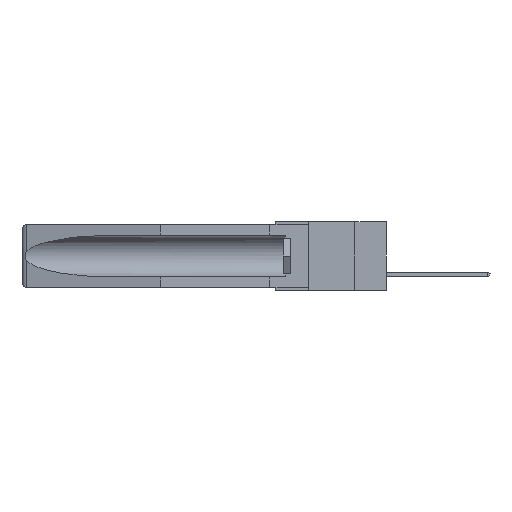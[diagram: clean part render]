
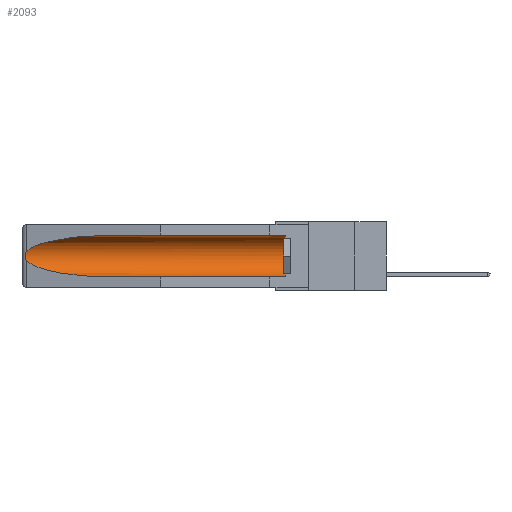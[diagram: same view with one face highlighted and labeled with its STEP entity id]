
A CAD part, left-side view. The second image highlights one B-rep face of the part: STEP entity #2093.
In plain terms, the highlighted cylindrical face has radius 2.857 mm (diameter 5.715 mm), a partial arc.
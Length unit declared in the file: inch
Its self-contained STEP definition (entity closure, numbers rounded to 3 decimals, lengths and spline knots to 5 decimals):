
#7 = CARTESIAN_POINT ( 'NONE',  ( 0.155, 0.126, -0.284 ) ) ;
#338 = CARTESIAN_POINT ( 'NONE',  ( 0.26655, 1.53094, -0.18657 ) ) ;
#1060 = ORIENTED_EDGE ( 'NONE', *, *, #14744, .T. ) ;
#1366 = CARTESIAN_POINT ( 'NONE',  ( 0.155, -0.30754, -0.284 ) ) ;
#1435 = CYLINDRICAL_SURFACE ( 'NONE', #15968, 0.1125 ) ;
#1681 = CARTESIAN_POINT ( 'NONE',  ( 0.155, 0.126, -0.1715 ) ) ;
#1811 = CARTESIAN_POINT ( 'NONE',  ( 0.155, -0.30754, -0.059 ) ) ;
#2093 = ADVANCED_FACE ( 'NONE', ( #4897 ), #1435, .F. ) ;
#2666 = VERTEX_POINT ( 'NONE', #25643 ) ;
#3251 = CARTESIAN_POINT ( 'NONE',  ( 0.21114, 1.30732, -0.059 ) ) ;
#3827 = DIRECTION ( 'NONE',  ( 0., 1., 0. ) ) ;
#3974 = CARTESIAN_POINT ( 'NONE',  ( 0.21114, 1.30732, -0.284 ) ) ;
#4140 = CARTESIAN_POINT ( 'NONE',  ( 0.2675, 1.53308, -0.17534 ) ) ;
#4897 = FACE_OUTER_BOUND ( 'NONE', #23598, .T. ) ;
#5046 = CARTESIAN_POINT ( 'NONE',  ( 0.155, -0.30754, -0.1715 ) ) ;
#5417 = VERTEX_POINT ( 'NONE', #7 ) ;
#7285 = ORIENTED_EDGE ( 'NONE', *, *, #19025, .T. ) ;
#8301 = CARTESIAN_POINT ( 'NONE',  ( 0.2673, 1.53269, -0.17917 ) ) ;
#8381 = CARTESIAN_POINT ( 'NONE',  ( 0.26654, 1.53092, -0.15636 ) ) ;
#8809 = EDGE_CURVE ( 'NONE', #5417, #25534, #17267, .T. ) ;
#8903 =( BOUNDED_CURVE ( )  B_SPLINE_CURVE ( 3, ( #23864, #11619, #3974, #10264 ),
 .UNSPECIFIED., .F., .F. ) 
 B_SPLINE_CURVE_WITH_KNOTS ( ( 4, 4 ),
 ( 0.1948, 1.5708 ),
 .UNSPECIFIED. ) 
 CURVE ( )  GEOMETRIC_REPRESENTATION_ITEM ( )  RATIONAL_B_SPLINE_CURVE ( ( 1., 0.848, 0.848, 1. ) ) 
 REPRESENTATION_ITEM ( '' )  );
#9391 = B_SPLINE_CURVE_WITH_KNOTS ( 'NONE', 3,
 ( #24817, #22938, #8381, #22679, #12441, #4140, #8301, #338, #20899, #10344 ),
 .UNSPECIFIED., .F., .F.,
 ( 4, 2, 2, 2, 4 ),
 ( 0., 0.00029, 0.00058, 0.00087, 0.00117 ),
 .UNSPECIFIED. ) ;
#9770 = CARTESIAN_POINT ( 'NONE',  ( 0.155, 0.126, -0.059 ) ) ;
#10205 =( BOUNDED_CURVE ( )  B_SPLINE_CURVE ( 3, ( #15561, #3251, #25621, #25446 ),
 .UNSPECIFIED., .F., .T. ) 
 B_SPLINE_CURVE_WITH_KNOTS ( ( 4, 4 ),
 ( 4.71239, 6.08839 ),
 .UNSPECIFIED. ) 
 CURVE ( )  GEOMETRIC_REPRESENTATION_ITEM ( )  RATIONAL_B_SPLINE_CURVE ( ( 1., 0.848, 0.848, 1. ) ) 
 REPRESENTATION_ITEM ( '' )  );
#10264 = CARTESIAN_POINT ( 'NONE',  ( 0.155, 1.07973, -0.284 ) ) ;
#10344 = CARTESIAN_POINT ( 'NONE',  ( 0.26537, 1.52718, -0.19328 ) ) ;
#10730 = VECTOR ( 'NONE', #3827, 39.37008 ) ;
#11619 = CARTESIAN_POINT ( 'NONE',  ( 0.25451, 1.48313, -0.24835 ) ) ;
#11975 = DIRECTION ( 'NONE',  ( 0., 1., 0. ) ) ;
#12441 = CARTESIAN_POINT ( 'NONE',  ( 0.2675, 1.53308, -0.16763 ) ) ;
#12499 = VERTEX_POINT ( 'NONE', #17276 ) ;
#13104 = EDGE_CURVE ( 'NONE', #5417, #16220, #15054, .T. ) ;
#13643 = ORIENTED_EDGE ( 'NONE', *, *, #16625, .T. ) ;
#13783 = VECTOR ( 'NONE', #25931, 39.37008 ) ;
#14066 = DIRECTION ( 'NONE',  ( 0., -1., 0. ) ) ;
#14294 = ORIENTED_EDGE ( 'NONE', *, *, #16226, .T. ) ;
#14310 = LINE ( 'NONE', #1811, #10730 ) ;
#14687 = CARTESIAN_POINT ( 'NONE',  ( 0.155, 1.07973, -0.284 ) ) ;
#14744 = EDGE_CURVE ( 'NONE', #2666, #25534, #8903, .T. ) ;
#15054 = CIRCLE ( 'NONE', #20045, 0.1125 ) ;
#15129 = ORIENTED_EDGE ( 'NONE', *, *, #8809, .F. ) ;
#15561 = CARTESIAN_POINT ( 'NONE',  ( 0.155, 1.07973, -0.059 ) ) ;
#15968 = AXIS2_PLACEMENT_3D ( 'NONE', #5046, #11975, #18075 ) ;
#16059 = VERTEX_POINT ( 'NONE', #21824 ) ;
#16220 = VERTEX_POINT ( 'NONE', #9770 ) ;
#16226 = EDGE_CURVE ( 'NONE', #16220, #16059, #14310, .T. ) ;
#16625 = EDGE_CURVE ( 'NONE', #16059, #12499, #10205, .T. ) ;
#17267 = LINE ( 'NONE', #1366, #13783 ) ;
#17276 = CARTESIAN_POINT ( 'NONE',  ( 0.26537, 1.52718, -0.14972 ) ) ;
#18075 = DIRECTION ( 'NONE',  ( 0., 0., 1. ) ) ;
#19025 = EDGE_CURVE ( 'NONE', #12499, #2666, #9391, .T. ) ;
#20045 = AXIS2_PLACEMENT_3D ( 'NONE', #1681, #14066, #24368 ) ;
#20163 = ORIENTED_EDGE ( 'NONE', *, *, #13104, .T. ) ;
#20899 = CARTESIAN_POINT ( 'NONE',  ( 0.26597, 1.5296, -0.19026 ) ) ;
#21824 = CARTESIAN_POINT ( 'NONE',  ( 0.155, 1.07973, -0.059 ) ) ;
#22679 = CARTESIAN_POINT ( 'NONE',  ( 0.2673, 1.5327, -0.16383 ) ) ;
#22938 = CARTESIAN_POINT ( 'NONE',  ( 0.26597, 1.52961, -0.15275 ) ) ;
#23598 = EDGE_LOOP ( 'NONE', ( #13643, #7285, #1060, #15129, #20163, #14294 ) ) ;
#23864 = CARTESIAN_POINT ( 'NONE',  ( 0.26537, 1.52718, -0.19328 ) ) ;
#24368 = DIRECTION ( 'NONE',  ( 0., 0., 1. ) ) ;
#24817 = CARTESIAN_POINT ( 'NONE',  ( 0.26537, 1.52718, -0.14972 ) ) ;
#25446 = CARTESIAN_POINT ( 'NONE',  ( 0.26537, 1.52718, -0.14972 ) ) ;
#25534 = VERTEX_POINT ( 'NONE', #14687 ) ;
#25621 = CARTESIAN_POINT ( 'NONE',  ( 0.25451, 1.48313, -0.09465 ) ) ;
#25643 = CARTESIAN_POINT ( 'NONE',  ( 0.26537, 1.52718, -0.19328 ) ) ;
#25931 = DIRECTION ( 'NONE',  ( 0., 1., 0. ) ) ;
